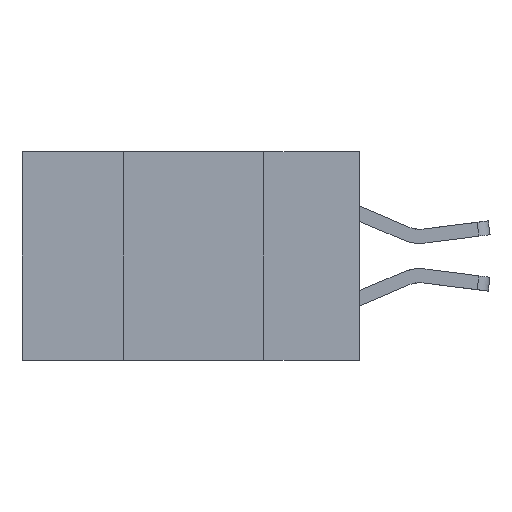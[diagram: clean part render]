
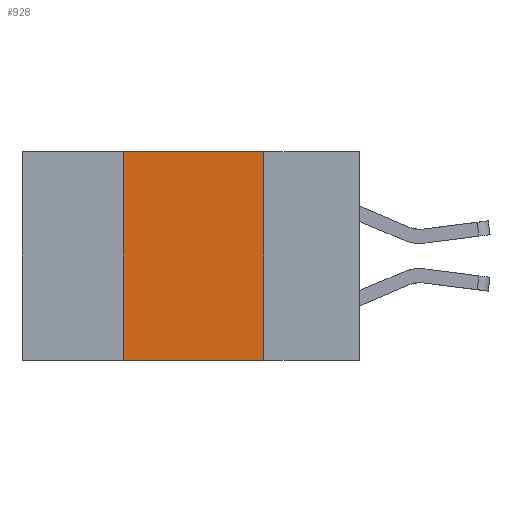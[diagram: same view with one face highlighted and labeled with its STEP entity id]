
A CAD part, left-side view. The second image highlights one B-rep face of the part: STEP entity #928.
In plain terms, the highlighted planar face has unit normal (-1, 0, 0).
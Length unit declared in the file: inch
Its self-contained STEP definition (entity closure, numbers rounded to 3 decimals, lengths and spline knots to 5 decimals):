
#928 = ADVANCED_FACE ( 'NONE', ( #7448 ), #5461, .F. ) ;
#1143 = VECTOR ( 'NONE', #12560, 39.37008 ) ;
#1185 = EDGE_LOOP ( 'NONE', ( #10977, #11289, #3586, #11618 ) ) ;
#1298 = EDGE_CURVE ( 'NONE', #13140, #12815, #1703, .T. ) ;
#1703 = LINE ( 'NONE', #11535, #12186 ) ;
#1943 = CARTESIAN_POINT ( 'NONE',  ( 0., 0.6, -0.37 ) ) ;
#1975 = DIRECTION ( 'NONE',  ( 0., -1., 0. ) ) ;
#2319 = EDGE_CURVE ( 'NONE', #13140, #6045, #6781, .T. ) ;
#3586 = ORIENTED_EDGE ( 'NONE', *, *, #1298, .F. ) ;
#4402 = DIRECTION ( 'NONE',  ( 0., -1., 0. ) ) ;
#4473 = LINE ( 'NONE', #11438, #9802 ) ;
#5283 = DIRECTION ( 'NONE',  ( 0., 0., -1. ) ) ;
#5381 = DIRECTION ( 'NONE',  ( 1., 0., 0. ) ) ;
#5420 = LINE ( 'NONE', #6505, #1143 ) ;
#5461 = PLANE ( 'NONE',  #10947 ) ;
#5528 = CARTESIAN_POINT ( 'NONE',  ( 0., 0.6, 0. ) ) ;
#6024 = VERTEX_POINT ( 'NONE', #9715 ) ;
#6045 = VERTEX_POINT ( 'NONE', #8743 ) ;
#6491 = EDGE_CURVE ( 'NONE', #12815, #6024, #4473, .T. ) ;
#6505 = CARTESIAN_POINT ( 'NONE',  ( 0., 0.17, 0. ) ) ;
#6781 = LINE ( 'NONE', #1943, #11844 ) ;
#7448 = FACE_OUTER_BOUND ( 'NONE', #1185, .T. ) ;
#7894 = CARTESIAN_POINT ( 'NONE',  ( 0., 0.42, -0.37 ) ) ;
#8743 = CARTESIAN_POINT ( 'NONE',  ( 0., 0.17, -0.37 ) ) ;
#9715 = CARTESIAN_POINT ( 'NONE',  ( 0., 0.17, 0. ) ) ;
#9802 = VECTOR ( 'NONE', #4402, 39.37008 ) ;
#10947 = AXIS2_PLACEMENT_3D ( 'NONE', #5528, #5381, #5283 ) ;
#10977 = ORIENTED_EDGE ( 'NONE', *, *, #11080, .F. ) ;
#11080 = EDGE_CURVE ( 'NONE', #6024, #6045, #5420, .T. ) ;
#11289 = ORIENTED_EDGE ( 'NONE', *, *, #6491, .F. ) ;
#11438 = CARTESIAN_POINT ( 'NONE',  ( 0., 0.6, 0. ) ) ;
#11467 = DIRECTION ( 'NONE',  ( 0., 0., 1. ) ) ;
#11535 = CARTESIAN_POINT ( 'NONE',  ( 0., 0.42, 0. ) ) ;
#11618 = ORIENTED_EDGE ( 'NONE', *, *, #2319, .T. ) ;
#11844 = VECTOR ( 'NONE', #1975, 39.37008 ) ;
#12186 = VECTOR ( 'NONE', #11467, 39.37008 ) ;
#12477 = CARTESIAN_POINT ( 'NONE',  ( 0., 0.42, 0. ) ) ;
#12560 = DIRECTION ( 'NONE',  ( 0., 0., -1. ) ) ;
#12815 = VERTEX_POINT ( 'NONE', #12477 ) ;
#13140 = VERTEX_POINT ( 'NONE', #7894 ) ;
